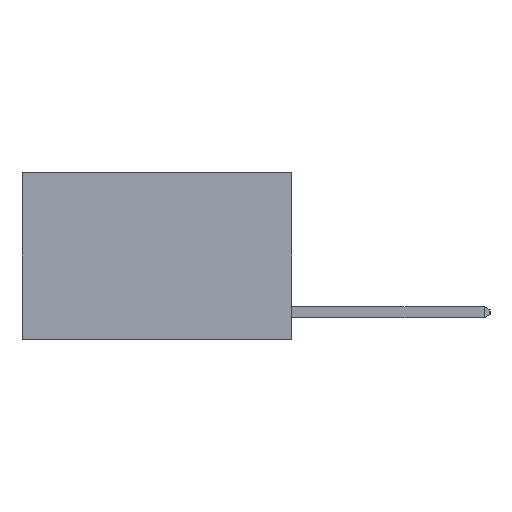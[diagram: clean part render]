
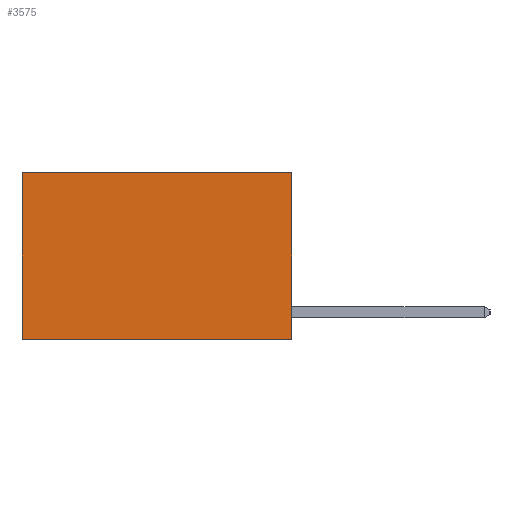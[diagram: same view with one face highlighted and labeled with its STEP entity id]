
A CAD part, left-side view. The second image highlights one B-rep face of the part: STEP entity #3575.
In plain terms, the highlighted planar face has unit normal (-1, 0, 0).
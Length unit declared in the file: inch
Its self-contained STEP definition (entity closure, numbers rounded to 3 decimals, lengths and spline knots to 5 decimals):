
#290 = LINE ( 'NONE', #6996, #8892 ) ;
#559 = PLANE ( 'NONE',  #4219 ) ;
#879 = ORIENTED_EDGE ( 'NONE', *, *, #7886, .T. ) ;
#1409 = DIRECTION ( 'NONE',  ( 1., 0., 0. ) ) ;
#2037 = VERTEX_POINT ( 'NONE', #10451 ) ;
#2197 = CARTESIAN_POINT ( 'NONE',  ( 0.2625, 0.6, 0. ) ) ;
#2666 = CARTESIAN_POINT ( 'NONE',  ( 0.2625, 0., -0.37 ) ) ;
#3293 = EDGE_CURVE ( 'NONE', #3364, #9117, #290, .T. ) ;
#3364 = VERTEX_POINT ( 'NONE', #5477 ) ;
#3575 = ADVANCED_FACE ( 'NONE', ( #4738 ), #559, .F. ) ;
#3582 = LINE ( 'NONE', #8048, #4332 ) ;
#3974 = LINE ( 'NONE', #2197, #8059 ) ;
#4219 = AXIS2_PLACEMENT_3D ( 'NONE', #6512, #1409, #7293 ) ;
#4247 = EDGE_CURVE ( 'NONE', #3364, #2037, #7374, .T. ) ;
#4332 = VECTOR ( 'NONE', #10459, 39.37008 ) ;
#4400 = ORIENTED_EDGE ( 'NONE', *, *, #4604, .F. ) ;
#4571 = ORIENTED_EDGE ( 'NONE', *, *, #3293, .F. ) ;
#4604 = EDGE_CURVE ( 'NONE', #9117, #7057, #3582, .T. ) ;
#4738 = FACE_OUTER_BOUND ( 'NONE', #10166, .T. ) ;
#5316 = CARTESIAN_POINT ( 'NONE',  ( 0.2625, 0., 0. ) ) ;
#5477 = CARTESIAN_POINT ( 'NONE',  ( 0.2625, 0., 0. ) ) ;
#6302 = CARTESIAN_POINT ( 'NONE',  ( 0.2625, 0.6, -0.37 ) ) ;
#6512 = CARTESIAN_POINT ( 'NONE',  ( 0.2625, 0., 0. ) ) ;
#6681 = ORIENTED_EDGE ( 'NONE', *, *, #4247, .T. ) ;
#6996 = CARTESIAN_POINT ( 'NONE',  ( 0.2625, 0., 0. ) ) ;
#7057 = VERTEX_POINT ( 'NONE', #6302 ) ;
#7293 = DIRECTION ( 'NONE',  ( 0., 0., -1. ) ) ;
#7374 = LINE ( 'NONE', #5316, #9268 ) ;
#7886 = EDGE_CURVE ( 'NONE', #2037, #7057, #3974, .T. ) ;
#8048 = CARTESIAN_POINT ( 'NONE',  ( 0.2625, 0., -0.37 ) ) ;
#8059 = VECTOR ( 'NONE', #8832, 39.37008 ) ;
#8832 = DIRECTION ( 'NONE',  ( 0., 0., -1. ) ) ;
#8892 = VECTOR ( 'NONE', #9407, 39.37008 ) ;
#9117 = VERTEX_POINT ( 'NONE', #2666 ) ;
#9268 = VECTOR ( 'NONE', #10121, 39.37008 ) ;
#9407 = DIRECTION ( 'NONE',  ( 0., 0., -1. ) ) ;
#10121 = DIRECTION ( 'NONE',  ( 0., 1., 0. ) ) ;
#10166 = EDGE_LOOP ( 'NONE', ( #879, #4400, #4571, #6681 ) ) ;
#10451 = CARTESIAN_POINT ( 'NONE',  ( 0.2625, 0.6, 0. ) ) ;
#10459 = DIRECTION ( 'NONE',  ( 0., 1., 0. ) ) ;
